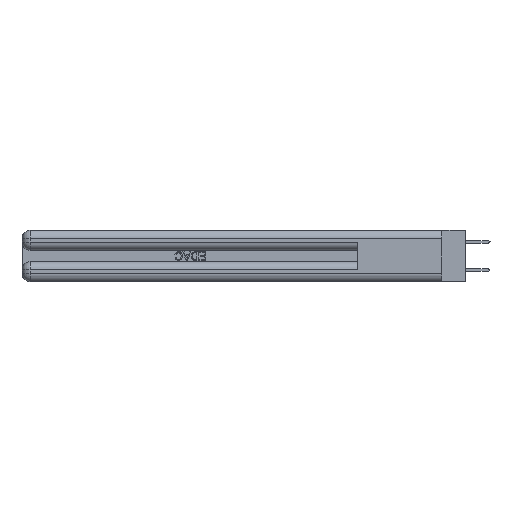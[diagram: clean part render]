
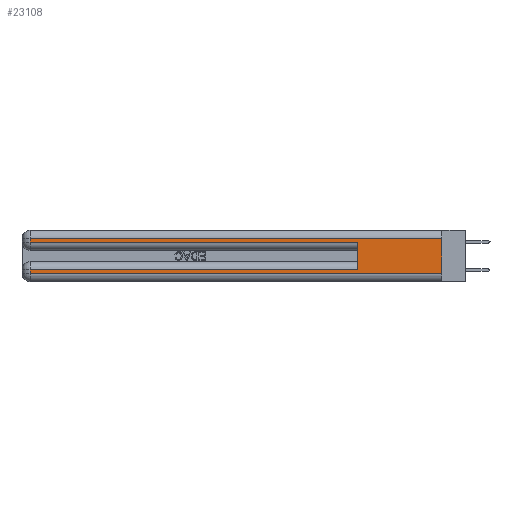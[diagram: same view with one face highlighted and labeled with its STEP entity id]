
A CAD part, left-side view. The second image highlights one B-rep face of the part: STEP entity #23108.
In plain terms, the highlighted planar face has unit normal (-1, 0, 0).
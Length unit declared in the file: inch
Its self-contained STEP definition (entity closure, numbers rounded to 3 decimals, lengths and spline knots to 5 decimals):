
#149 = VERTEX_POINT ( 'NONE', #12529 ) ;
#555 = EDGE_CURVE ( 'NONE', #22678, #27113, #14656, .T. ) ;
#652 = EDGE_CURVE ( 'NONE', #4996, #13514, #20034, .T. ) ;
#785 = CARTESIAN_POINT ( 'NONE',  ( 0., 0.6, 0.145 ) ) ;
#892 = LINE ( 'NONE', #35729, #25796 ) ;
#1046 = PLANE ( 'NONE',  #21138 ) ;
#1304 = VERTEX_POINT ( 'NONE', #24412 ) ;
#2138 = DIRECTION ( 'NONE',  ( 0., 0., -1. ) ) ;
#2427 = CARTESIAN_POINT ( 'NONE',  ( 0., 2.94, 0.285 ) ) ;
#3138 = LINE ( 'NONE', #22312, #35739 ) ;
#3300 = DIRECTION ( 'NONE',  ( 0., 0., 1. ) ) ;
#4996 = VERTEX_POINT ( 'NONE', #26625 ) ;
#5860 = ORIENTED_EDGE ( 'NONE', *, *, #9880, .F. ) ;
#8135 = DIRECTION ( 'NONE',  ( 0., -1., 0. ) ) ;
#9880 = EDGE_CURVE ( 'NONE', #22678, #13514, #12164, .T. ) ;
#11730 = VECTOR ( 'NONE', #24094, 39.37008 ) ;
#12164 = LINE ( 'NONE', #38737, #37986 ) ;
#12529 = CARTESIAN_POINT ( 'NONE',  ( 0., 0.6, 0.085 ) ) ;
#12706 = CARTESIAN_POINT ( 'NONE',  ( 0., 2.94, 0.37 ) ) ;
#13008 = LINE ( 'NONE', #20531, #19346 ) ;
#13514 = VERTEX_POINT ( 'NONE', #36984 ) ;
#14160 = VECTOR ( 'NONE', #39451, 39.37008 ) ;
#14633 = ORIENTED_EDGE ( 'NONE', *, *, #31177, .T. ) ;
#14656 = LINE ( 'NONE', #14668, #14160 ) ;
#14668 = CARTESIAN_POINT ( 'NONE',  ( 0., 0., 0.31 ) ) ;
#15363 = LINE ( 'NONE', #12706, #32919 ) ;
#16226 = VERTEX_POINT ( 'NONE', #2427 ) ;
#16258 = ORIENTED_EDGE ( 'NONE', *, *, #34127, .T. ) ;
#16362 = VERTEX_POINT ( 'NONE', #24316 ) ;
#19346 = VECTOR ( 'NONE', #8135, 39.37008 ) ;
#19361 = EDGE_CURVE ( 'NONE', #149, #16362, #24735, .T. ) ;
#19669 = DIRECTION ( 'NONE',  ( 0., 0., -1. ) ) ;
#19694 = CARTESIAN_POINT ( 'NONE',  ( 0., 2.94, 0.31 ) ) ;
#20034 = LINE ( 'NONE', #30068, #11730 ) ;
#20531 = CARTESIAN_POINT ( 'NONE',  ( 0., 0., 0.285 ) ) ;
#20981 = CARTESIAN_POINT ( 'NONE',  ( 0., 0., 0.31 ) ) ;
#21138 = AXIS2_PLACEMENT_3D ( 'NONE', #35380, #29928, #2138 ) ;
#22312 = CARTESIAN_POINT ( 'NONE',  ( 0., 2.94, 0.37 ) ) ;
#22678 = VERTEX_POINT ( 'NONE', #20981 ) ;
#23108 = ADVANCED_FACE ( 'NONE', ( #38140 ), #1046, .F. ) ;
#24094 = DIRECTION ( 'NONE',  ( 0., -1., 0. ) ) ;
#24316 = CARTESIAN_POINT ( 'NONE',  ( 0., 0.6, 0.285 ) ) ;
#24412 = CARTESIAN_POINT ( 'NONE',  ( 0., 2.94, 0.085 ) ) ;
#24735 = LINE ( 'NONE', #785, #26631 ) ;
#24918 = DIRECTION ( 'NONE',  ( 0., 0., -1. ) ) ;
#25796 = VECTOR ( 'NONE', #32865, 39.37008 ) ;
#26341 = ORIENTED_EDGE ( 'NONE', *, *, #19361, .F. ) ;
#26505 = EDGE_LOOP ( 'NONE', ( #5860, #27092, #16258, #36287, #26341, #14633, #27893, #31297 ) ) ;
#26625 = CARTESIAN_POINT ( 'NONE',  ( 0., 2.94, 0.06 ) ) ;
#26631 = VECTOR ( 'NONE', #3300, 39.37008 ) ;
#27092 = ORIENTED_EDGE ( 'NONE', *, *, #555, .T. ) ;
#27113 = VERTEX_POINT ( 'NONE', #19694 ) ;
#27893 = ORIENTED_EDGE ( 'NONE', *, *, #28648, .T. ) ;
#28485 = DIRECTION ( 'NONE',  ( 0., 0., -1. ) ) ;
#28648 = EDGE_CURVE ( 'NONE', #1304, #4996, #3138, .T. ) ;
#29928 = DIRECTION ( 'NONE',  ( 1., 0., 0. ) ) ;
#30068 = CARTESIAN_POINT ( 'NONE',  ( 0., 0., 0.06 ) ) ;
#31177 = EDGE_CURVE ( 'NONE', #149, #1304, #892, .T. ) ;
#31297 = ORIENTED_EDGE ( 'NONE', *, *, #652, .T. ) ;
#32865 = DIRECTION ( 'NONE',  ( 0., 1., 0. ) ) ;
#32919 = VECTOR ( 'NONE', #28485, 39.37008 ) ;
#34127 = EDGE_CURVE ( 'NONE', #27113, #16226, #15363, .T. ) ;
#35380 = CARTESIAN_POINT ( 'NONE',  ( 0., 0., 0.37 ) ) ;
#35729 = CARTESIAN_POINT ( 'NONE',  ( 0., 0., 0.085 ) ) ;
#35739 = VECTOR ( 'NONE', #24918, 39.37008 ) ;
#36287 = ORIENTED_EDGE ( 'NONE', *, *, #38093, .T. ) ;
#36984 = CARTESIAN_POINT ( 'NONE',  ( 0., 0., 0.06 ) ) ;
#37986 = VECTOR ( 'NONE', #19669, 39.37008 ) ;
#38093 = EDGE_CURVE ( 'NONE', #16226, #16362, #13008, .T. ) ;
#38140 = FACE_OUTER_BOUND ( 'NONE', #26505, .T. ) ;
#38737 = CARTESIAN_POINT ( 'NONE',  ( 0., 0., 0.37 ) ) ;
#39451 = DIRECTION ( 'NONE',  ( 0., 1., 0. ) ) ;
